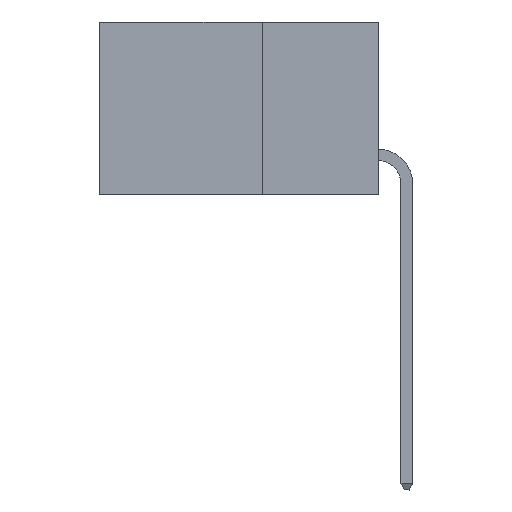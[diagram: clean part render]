
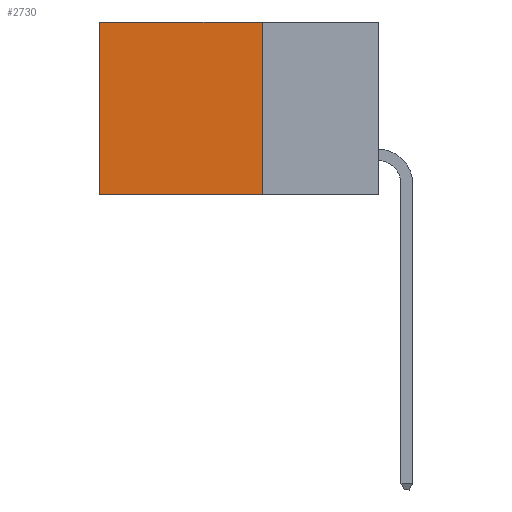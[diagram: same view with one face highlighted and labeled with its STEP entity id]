
A CAD part, left-side view. The second image highlights one B-rep face of the part: STEP entity #2730.
In plain terms, the highlighted planar face has unit normal (-1, 0, 0).
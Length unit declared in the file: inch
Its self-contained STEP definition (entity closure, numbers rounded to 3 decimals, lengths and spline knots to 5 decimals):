
#378 = CARTESIAN_POINT ( 'NONE',  ( 0.298, 0.25, 0. ) ) ;
#1572 = LINE ( 'NONE', #3893, #2200 ) ;
#2200 = VECTOR ( 'NONE', #3799, 39.37008 ) ;
#2730 = ADVANCED_FACE ( 'NONE', ( #8290 ), #20646, .F. ) ;
#2818 = EDGE_CURVE ( 'NONE', #18079, #17516, #1572, .T. ) ;
#3114 = EDGE_CURVE ( 'NONE', #4572, #18079, #13727, .T. ) ;
#3799 = DIRECTION ( 'NONE',  ( 0., 0., -1. ) ) ;
#3893 = CARTESIAN_POINT ( 'NONE',  ( 0.298, 0.6, 0. ) ) ;
#4572 = VERTEX_POINT ( 'NONE', #5175 ) ;
#5009 = EDGE_CURVE ( 'NONE', #4572, #18814, #22535, .T. ) ;
#5175 = CARTESIAN_POINT ( 'NONE',  ( 0.298, 0.25, 0. ) ) ;
#7080 = LINE ( 'NONE', #23251, #16263 ) ;
#7504 = EDGE_CURVE ( 'NONE', #18814, #17516, #7080, .T. ) ;
#7814 = CARTESIAN_POINT ( 'NONE',  ( 0.298, 0.25, -0.37 ) ) ;
#8290 = FACE_OUTER_BOUND ( 'NONE', #10068, .T. ) ;
#8384 = ORIENTED_EDGE ( 'NONE', *, *, #5009, .F. ) ;
#10068 = EDGE_LOOP ( 'NONE', ( #19582, #21610, #8384, #19385 ) ) ;
#13727 = LINE ( 'NONE', #378, #18042 ) ;
#13877 = DIRECTION ( 'NONE',  ( 0., 0., -1. ) ) ;
#14366 = AXIS2_PLACEMENT_3D ( 'NONE', #22278, #20550, #13877 ) ;
#16263 = VECTOR ( 'NONE', #20123, 39.37008 ) ;
#16594 = CARTESIAN_POINT ( 'NONE',  ( 0.298, 0.6, -0.37 ) ) ;
#17516 = VERTEX_POINT ( 'NONE', #16594 ) ;
#17735 = VECTOR ( 'NONE', #18196, 39.37008 ) ;
#18042 = VECTOR ( 'NONE', #23631, 39.37008 ) ;
#18079 = VERTEX_POINT ( 'NONE', #23704 ) ;
#18172 = CARTESIAN_POINT ( 'NONE',  ( 0.298, 0.25, 0. ) ) ;
#18196 = DIRECTION ( 'NONE',  ( 0., 0., -1. ) ) ;
#18814 = VERTEX_POINT ( 'NONE', #7814 ) ;
#19385 = ORIENTED_EDGE ( 'NONE', *, *, #3114, .T. ) ;
#19582 = ORIENTED_EDGE ( 'NONE', *, *, #2818, .T. ) ;
#20123 = DIRECTION ( 'NONE',  ( 0., 1., 0. ) ) ;
#20550 = DIRECTION ( 'NONE',  ( 1., 0., 0. ) ) ;
#20646 = PLANE ( 'NONE',  #14366 ) ;
#21610 = ORIENTED_EDGE ( 'NONE', *, *, #7504, .F. ) ;
#22278 = CARTESIAN_POINT ( 'NONE',  ( 0.298, 0.25, 0. ) ) ;
#22535 = LINE ( 'NONE', #18172, #17735 ) ;
#23251 = CARTESIAN_POINT ( 'NONE',  ( 0.298, 0.25, -0.37 ) ) ;
#23631 = DIRECTION ( 'NONE',  ( 0., 1., 0. ) ) ;
#23704 = CARTESIAN_POINT ( 'NONE',  ( 0.298, 0.6, 0. ) ) ;
